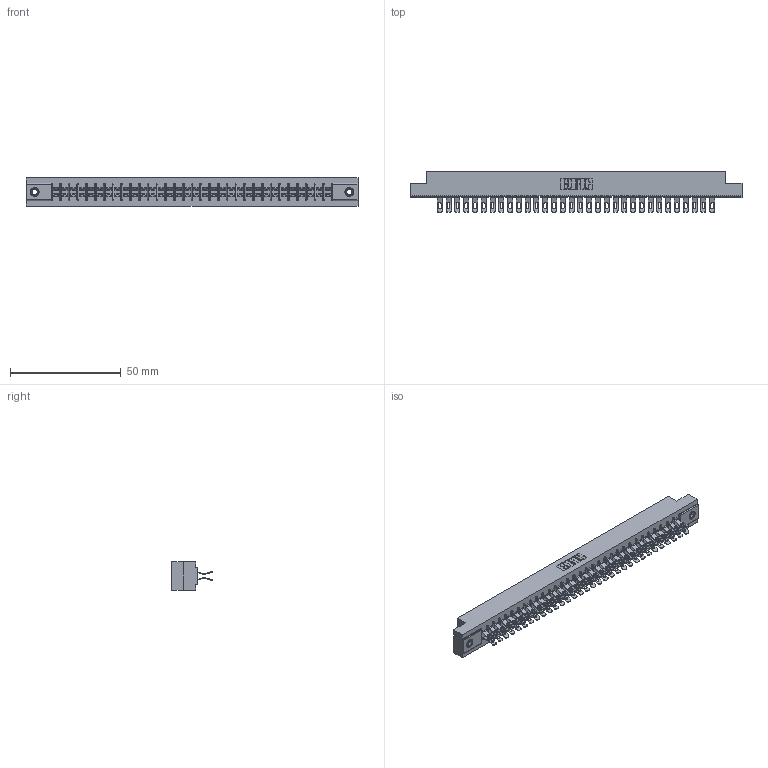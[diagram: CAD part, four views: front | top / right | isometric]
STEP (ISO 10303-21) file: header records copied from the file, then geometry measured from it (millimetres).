
FILE_DESCRIPTION (( 'STEP AP203' ), '1' );
FILE_NAME ('305-064-555-507.STEP', '2019-09-10T02:58:55', ( '' ), ( '' ), 'SwSTEP 2.0', 'SolidWorks 2016', '' );
FILE_SCHEMA (( 'CONFIG_CONTROL_DESIGN' ));
Length unit declared in the file: inch
Products named in the file (4): 305-290-001_555; 305 Part_.156 Dia; 345-250-001_345-250-005-103; 305-064-555-507
Assembly tree (67 placements, depth 2):
  305-064-555-507
    305 Part_.156 Dia
    305-290-001_555  x64
    345-250-001_345-250-005-103  x2
Bounding box: 149.81 x 18.41 x 12.7 mm (x, y, z)
Volume: 15301 mm3; surface area: 21186.8 mm2
Topology: 67 solids, 67 shells, 4400 faces, 13092 edges, 8548 vertices
Faces by surface type: plane 2148, cylinder 2108, sphere 128, cone 12, torus 4
Entity records: 37674 total; most frequent: CARTESIAN_POINT 6235, ORIENTED_EDGE 6172, DIRECTION 6044, EDGE_CURVE 3086, VECTOR 2462, LINE 2462, VERTEX_POINT 1966, AXIS2_PLACEMENT_3D 1791
